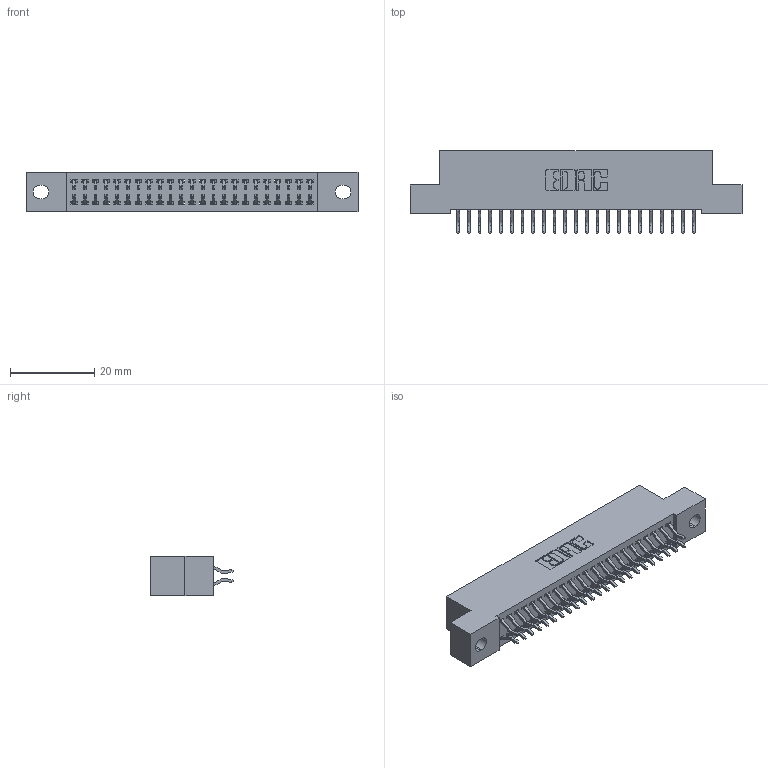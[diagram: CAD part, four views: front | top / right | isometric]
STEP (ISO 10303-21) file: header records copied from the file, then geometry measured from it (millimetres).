
FILE_DESCRIPTION (( 'STEP AP203' ), '1' );
FILE_NAME ('342-046-556-202.STEP', '2019-10-02T20:52:09', ( '' ), ( '' ), 'SwSTEP 2.0', 'SolidWorks 2016', '' );
FILE_SCHEMA (( 'CONFIG_CONTROL_DESIGN' ));
Length unit declared in the file: inch
Products named in the file (3): 342 Part_.128 Slot; 345-292-001_556 Tail; 342-046-556-202
Assembly tree (47 placements, depth 2):
  342-046-556-202
    342 Part_.128 Slot
    345-292-001_556 Tail  x46
Bounding box: 78.74 x 19.58 x 9.4 mm (x, y, z)
Volume: 6931.5 mm3; surface area: 10529.5 mm2
Topology: 47 solids, 47 shells, 2782 faces, 8269 edges, 5450 vertices
Faces by surface type: plane 1910, cylinder 872
Entity records: 17477 total; most frequent: CARTESIAN_POINT 2934, ORIENTED_EDGE 2858, DIRECTION 2529, EDGE_CURVE 1429, VECTOR 1293, LINE 1293, VERTEX_POINT 950, AXIS2_PLACEMENT_3D 618
